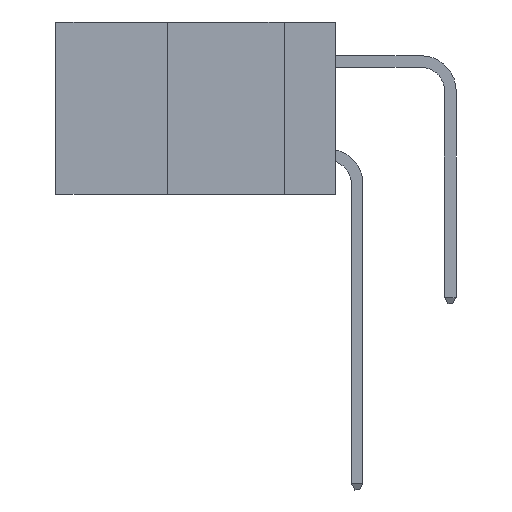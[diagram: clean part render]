
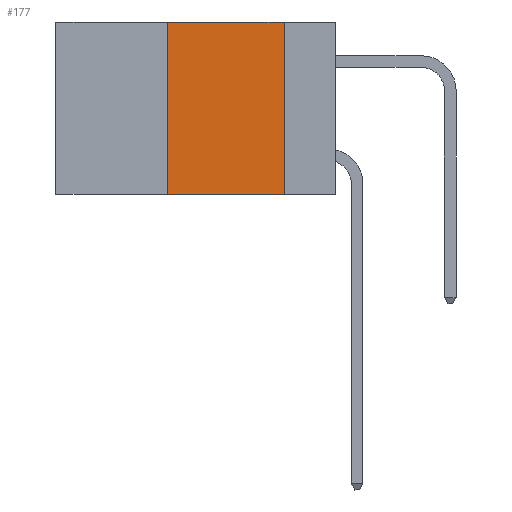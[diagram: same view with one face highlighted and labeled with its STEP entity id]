
A CAD part, left-side view. The second image highlights one B-rep face of the part: STEP entity #177.
In plain terms, the highlighted planar face has unit normal (-1, 0, 0).
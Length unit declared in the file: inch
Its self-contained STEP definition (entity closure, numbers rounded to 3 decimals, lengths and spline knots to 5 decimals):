
#162 = LINE ( 'NONE', #8718, #4231 ) ;
#177 = ADVANCED_FACE ( 'NONE', ( #12637 ), #8249, .F. ) ;
#654 = AXIS2_PLACEMENT_3D ( 'NONE', #8525, #841, #3325 ) ;
#841 = DIRECTION ( 'NONE',  ( 1., 0., 0. ) ) ;
#1085 = VECTOR ( 'NONE', #2175, 39.37008 ) ;
#1220 = CARTESIAN_POINT ( 'NONE',  ( 0., 0.36, 0. ) ) ;
#1764 = ORIENTED_EDGE ( 'NONE', *, *, #9758, .F. ) ;
#1832 = DIRECTION ( 'NONE',  ( 0., 0., 1. ) ) ;
#2139 = CARTESIAN_POINT ( 'NONE',  ( 0., 0.11, -0.37 ) ) ;
#2175 = DIRECTION ( 'NONE',  ( 0., -1., 0. ) ) ;
#2189 = LINE ( 'NONE', #10835, #11238 ) ;
#2206 = EDGE_CURVE ( 'NONE', #13316, #4095, #7645, .T. ) ;
#2964 = VERTEX_POINT ( 'NONE', #7433 ) ;
#3325 = DIRECTION ( 'NONE',  ( 0., 0., -1. ) ) ;
#4095 = VERTEX_POINT ( 'NONE', #6657 ) ;
#4231 = VECTOR ( 'NONE', #7416, 39.37008 ) ;
#6316 = ORIENTED_EDGE ( 'NONE', *, *, #15594, .F. ) ;
#6657 = CARTESIAN_POINT ( 'NONE',  ( 0., 0.11, 0. ) ) ;
#7416 = DIRECTION ( 'NONE',  ( 0., 0., -1. ) ) ;
#7433 = CARTESIAN_POINT ( 'NONE',  ( 0., 0.36, -0.37 ) ) ;
#7645 = LINE ( 'NONE', #9166, #1085 ) ;
#8249 = PLANE ( 'NONE',  #654 ) ;
#8403 = EDGE_LOOP ( 'NONE', ( #6316, #13906, #1764, #13555 ) ) ;
#8437 = DIRECTION ( 'NONE',  ( 0., -1., 0. ) ) ;
#8525 = CARTESIAN_POINT ( 'NONE',  ( 0., 0.6, 0. ) ) ;
#8718 = CARTESIAN_POINT ( 'NONE',  ( 0., 0.11, 0. ) ) ;
#9166 = CARTESIAN_POINT ( 'NONE',  ( 0., 0.6, 0. ) ) ;
#9758 = EDGE_CURVE ( 'NONE', #2964, #13316, #10610, .T. ) ;
#10108 = VERTEX_POINT ( 'NONE', #2139 ) ;
#10610 = LINE ( 'NONE', #15342, #15361 ) ;
#10835 = CARTESIAN_POINT ( 'NONE',  ( 0., 0.6, -0.37 ) ) ;
#11238 = VECTOR ( 'NONE', #8437, 39.37008 ) ;
#12637 = FACE_OUTER_BOUND ( 'NONE', #8403, .T. ) ;
#12670 = EDGE_CURVE ( 'NONE', #2964, #10108, #2189, .T. ) ;
#13316 = VERTEX_POINT ( 'NONE', #1220 ) ;
#13555 = ORIENTED_EDGE ( 'NONE', *, *, #12670, .T. ) ;
#13906 = ORIENTED_EDGE ( 'NONE', *, *, #2206, .F. ) ;
#15342 = CARTESIAN_POINT ( 'NONE',  ( 0., 0.36, 0. ) ) ;
#15361 = VECTOR ( 'NONE', #1832, 39.37008 ) ;
#15594 = EDGE_CURVE ( 'NONE', #4095, #10108, #162, .T. ) ;
